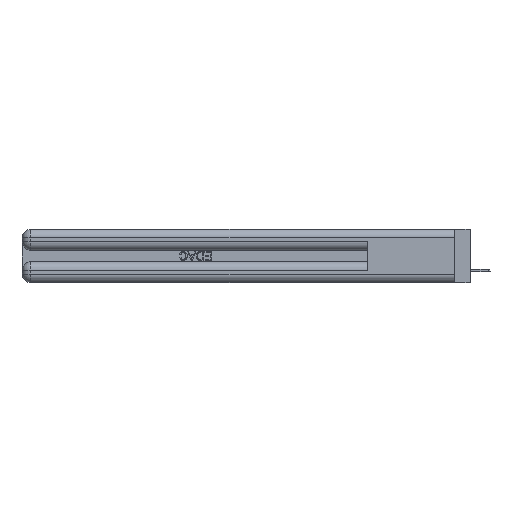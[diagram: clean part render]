
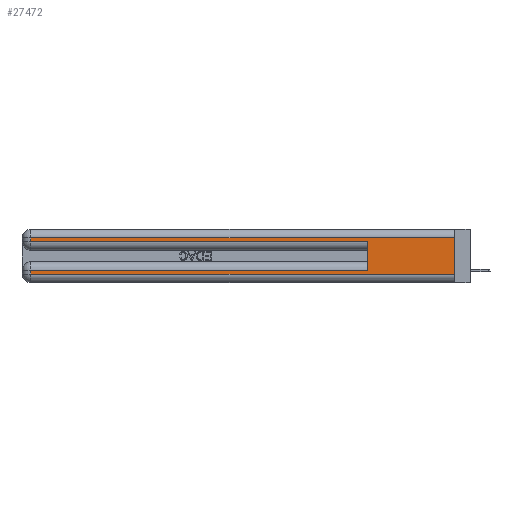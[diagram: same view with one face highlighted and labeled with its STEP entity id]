
A CAD part, left-side view. The second image highlights one B-rep face of the part: STEP entity #27472.
In plain terms, the highlighted planar face has unit normal (-1, 0, 0).
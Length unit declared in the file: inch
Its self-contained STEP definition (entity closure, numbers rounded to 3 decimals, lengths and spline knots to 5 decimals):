
#895 = VECTOR ( 'NONE', #19780, 39.37008 ) ;
#1047 = ORIENTED_EDGE ( 'NONE', *, *, #31443, .T. ) ;
#3079 = EDGE_CURVE ( 'NONE', #33003, #45909, #7330, .T. ) ;
#3322 = CARTESIAN_POINT ( 'NONE',  ( 0., 0., 0.06 ) ) ;
#3330 = LINE ( 'NONE', #27458, #3828 ) ;
#3428 = DIRECTION ( 'NONE',  ( 0., 0., -1. ) ) ;
#3725 = VERTEX_POINT ( 'NONE', #32618 ) ;
#3828 = VECTOR ( 'NONE', #30587, 39.37008 ) ;
#5389 = CARTESIAN_POINT ( 'NONE',  ( 0., 2.94, 0.085 ) ) ;
#6304 = ORIENTED_EDGE ( 'NONE', *, *, #12869, .T. ) ;
#7330 = LINE ( 'NONE', #39616, #14116 ) ;
#7665 = AXIS2_PLACEMENT_3D ( 'NONE', #33950, #45514, #49954 ) ;
#8356 = EDGE_CURVE ( 'NONE', #51141, #50209, #3330, .T. ) ;
#11301 = DIRECTION ( 'NONE',  ( 0., 0., -1. ) ) ;
#12869 = EDGE_CURVE ( 'NONE', #3725, #14491, #44399, .T. ) ;
#13776 = ORIENTED_EDGE ( 'NONE', *, *, #40428, .T. ) ;
#14116 = VECTOR ( 'NONE', #29960, 39.37008 ) ;
#14228 = PLANE ( 'NONE',  #7665 ) ;
#14491 = VERTEX_POINT ( 'NONE', #43407 ) ;
#14912 = CARTESIAN_POINT ( 'NONE',  ( 0., 2.94, 0.285 ) ) ;
#15884 = ORIENTED_EDGE ( 'NONE', *, *, #8356, .F. ) ;
#16367 = LINE ( 'NONE', #40820, #26204 ) ;
#17146 = FACE_OUTER_BOUND ( 'NONE', #21923, .T. ) ;
#18856 = LINE ( 'NONE', #22812, #51561 ) ;
#19456 = CARTESIAN_POINT ( 'NONE',  ( 0., 0., 0.37 ) ) ;
#19780 = DIRECTION ( 'NONE',  ( 0., -1., 0. ) ) ;
#20290 = VECTOR ( 'NONE', #11301, 39.37008 ) ;
#21923 = EDGE_LOOP ( 'NONE', ( #30411, #51046, #40318, #13776, #15884, #44067, #1047, #6304 ) ) ;
#22812 = CARTESIAN_POINT ( 'NONE',  ( 0., 2.94, 0.37 ) ) ;
#24373 = CARTESIAN_POINT ( 'NONE',  ( 0., 2.94, 0.31 ) ) ;
#24606 = VECTOR ( 'NONE', #42029, 39.37008 ) ;
#26204 = VECTOR ( 'NONE', #32410, 39.37008 ) ;
#27437 = LINE ( 'NONE', #47078, #895 ) ;
#27458 = CARTESIAN_POINT ( 'NONE',  ( 0., 0.6, 0.145 ) ) ;
#27472 = ADVANCED_FACE ( 'NONE', ( #17146 ), #14228, .F. ) ;
#27874 = CARTESIAN_POINT ( 'NONE',  ( 0., 0.6, 0.285 ) ) ;
#28231 = VERTEX_POINT ( 'NONE', #44550 ) ;
#28528 = EDGE_CURVE ( 'NONE', #51141, #40405, #16367, .T. ) ;
#29960 = DIRECTION ( 'NONE',  ( 0., 0., -1. ) ) ;
#30411 = ORIENTED_EDGE ( 'NONE', *, *, #48945, .F. ) ;
#30587 = DIRECTION ( 'NONE',  ( 0., 0., 1. ) ) ;
#31020 = VECTOR ( 'NONE', #32570, 39.37008 ) ;
#31443 = EDGE_CURVE ( 'NONE', #40405, #3725, #18856, .T. ) ;
#32410 = DIRECTION ( 'NONE',  ( 0., 1., 0. ) ) ;
#32570 = DIRECTION ( 'NONE',  ( 0., -1., 0. ) ) ;
#32618 = CARTESIAN_POINT ( 'NONE',  ( 0., 2.94, 0.06 ) ) ;
#33003 = VERTEX_POINT ( 'NONE', #24373 ) ;
#33950 = CARTESIAN_POINT ( 'NONE',  ( 0., 0., 0.37 ) ) ;
#39616 = CARTESIAN_POINT ( 'NONE',  ( 0., 2.94, 0.37 ) ) ;
#40318 = ORIENTED_EDGE ( 'NONE', *, *, #3079, .T. ) ;
#40405 = VERTEX_POINT ( 'NONE', #5389 ) ;
#40428 = EDGE_CURVE ( 'NONE', #45909, #50209, #27437, .T. ) ;
#40820 = CARTESIAN_POINT ( 'NONE',  ( 0., 0., 0.085 ) ) ;
#41448 = CARTESIAN_POINT ( 'NONE',  ( 0., 0.6, 0.085 ) ) ;
#42029 = DIRECTION ( 'NONE',  ( 0., 1., 0. ) ) ;
#43407 = CARTESIAN_POINT ( 'NONE',  ( 0., 0., 0.06 ) ) ;
#44067 = ORIENTED_EDGE ( 'NONE', *, *, #28528, .T. ) ;
#44399 = LINE ( 'NONE', #3322, #31020 ) ;
#44550 = CARTESIAN_POINT ( 'NONE',  ( 0., 0., 0.31 ) ) ;
#44733 = CARTESIAN_POINT ( 'NONE',  ( 0., 0., 0.31 ) ) ;
#45004 = LINE ( 'NONE', #44733, #24606 ) ;
#45514 = DIRECTION ( 'NONE',  ( 1., 0., 0. ) ) ;
#45909 = VERTEX_POINT ( 'NONE', #14912 ) ;
#47078 = CARTESIAN_POINT ( 'NONE',  ( 0., 0., 0.285 ) ) ;
#47265 = LINE ( 'NONE', #19456, #20290 ) ;
#48945 = EDGE_CURVE ( 'NONE', #28231, #14491, #47265, .T. ) ;
#49954 = DIRECTION ( 'NONE',  ( 0., 0., -1. ) ) ;
#50209 = VERTEX_POINT ( 'NONE', #27874 ) ;
#50744 = EDGE_CURVE ( 'NONE', #28231, #33003, #45004, .T. ) ;
#51046 = ORIENTED_EDGE ( 'NONE', *, *, #50744, .T. ) ;
#51141 = VERTEX_POINT ( 'NONE', #41448 ) ;
#51561 = VECTOR ( 'NONE', #3428, 39.37008 ) ;
